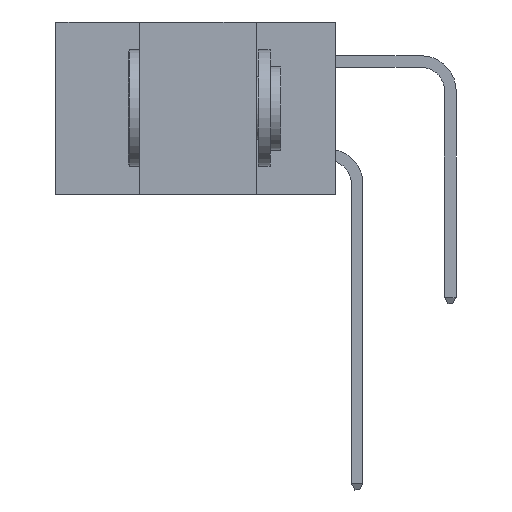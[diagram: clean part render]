
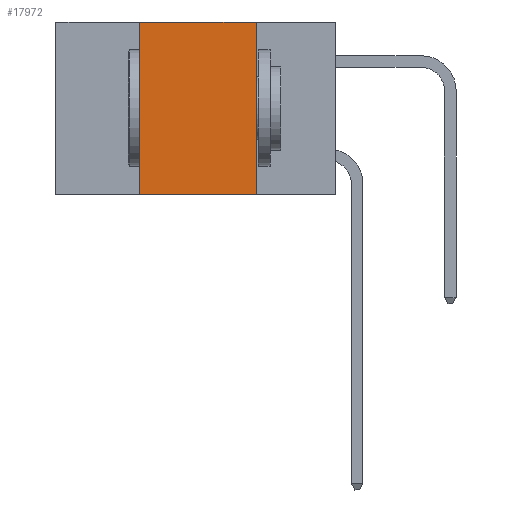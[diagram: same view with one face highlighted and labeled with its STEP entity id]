
A CAD part, left-side view. The second image highlights one B-rep face of the part: STEP entity #17972.
In plain terms, the highlighted planar face has unit normal (-1, 0, 0).
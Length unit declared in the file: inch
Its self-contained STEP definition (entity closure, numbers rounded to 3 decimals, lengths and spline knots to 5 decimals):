
#1088 = EDGE_CURVE ( 'NONE', #13339, #32797, #9101, .T. ) ;
#1753 = DIRECTION ( 'NONE',  ( 0., 0., 1. ) ) ;
#2459 = CARTESIAN_POINT ( 'NONE',  ( 0., 0.6, 0. ) ) ;
#3447 = AXIS2_PLACEMENT_3D ( 'NONE', #6194, #25549, #22922 ) ;
#5418 = VECTOR ( 'NONE', #20588, 39.37008 ) ;
#5605 = EDGE_CURVE ( 'NONE', #18324, #12103, #6282, .T. ) ;
#6194 = CARTESIAN_POINT ( 'NONE',  ( 0., 0.6, 0. ) ) ;
#6282 = LINE ( 'NONE', #19044, #5418 ) ;
#7973 = ORIENTED_EDGE ( 'NONE', *, *, #1088, .F. ) ;
#9101 = LINE ( 'NONE', #34495, #34748 ) ;
#10154 = CARTESIAN_POINT ( 'NONE',  ( 0., 0.17, 0. ) ) ;
#11293 = CARTESIAN_POINT ( 'NONE',  ( 0., 0.42, -0.37 ) ) ;
#11452 = EDGE_LOOP ( 'NONE', ( #32067, #30762, #7973, #21016 ) ) ;
#12103 = VERTEX_POINT ( 'NONE', #30234 ) ;
#13339 = VERTEX_POINT ( 'NONE', #11293 ) ;
#15178 = DIRECTION ( 'NONE',  ( 0., -1., 0. ) ) ;
#15244 = VECTOR ( 'NONE', #15178, 39.37008 ) ;
#17972 = ADVANCED_FACE ( 'NONE', ( #26193 ), #30683, .F. ) ;
#18324 = VERTEX_POINT ( 'NONE', #10154 ) ;
#19044 = CARTESIAN_POINT ( 'NONE',  ( 0., 0.17, 0. ) ) ;
#20588 = DIRECTION ( 'NONE',  ( 0., 0., -1. ) ) ;
#20861 = LINE ( 'NONE', #2459, #31932 ) ;
#21016 = ORIENTED_EDGE ( 'NONE', *, *, #34148, .T. ) ;
#22922 = DIRECTION ( 'NONE',  ( 0., 0., -1. ) ) ;
#24076 = DIRECTION ( 'NONE',  ( 0., -1., 0. ) ) ;
#25549 = DIRECTION ( 'NONE',  ( 1., 0., 0. ) ) ;
#26193 = FACE_OUTER_BOUND ( 'NONE', #11452, .T. ) ;
#27192 = EDGE_CURVE ( 'NONE', #32797, #18324, #20861, .T. ) ;
#30234 = CARTESIAN_POINT ( 'NONE',  ( 0., 0.17, -0.37 ) ) ;
#30683 = PLANE ( 'NONE',  #3447 ) ;
#30762 = ORIENTED_EDGE ( 'NONE', *, *, #27192, .F. ) ;
#31932 = VECTOR ( 'NONE', #24076, 39.37008 ) ;
#31948 = CARTESIAN_POINT ( 'NONE',  ( 0., 0.6, -0.37 ) ) ;
#32067 = ORIENTED_EDGE ( 'NONE', *, *, #5605, .F. ) ;
#32281 = LINE ( 'NONE', #31948, #15244 ) ;
#32797 = VERTEX_POINT ( 'NONE', #34342 ) ;
#34148 = EDGE_CURVE ( 'NONE', #13339, #12103, #32281, .T. ) ;
#34342 = CARTESIAN_POINT ( 'NONE',  ( 0., 0.42, 0. ) ) ;
#34495 = CARTESIAN_POINT ( 'NONE',  ( 0., 0.42, 0. ) ) ;
#34748 = VECTOR ( 'NONE', #1753, 39.37008 ) ;
